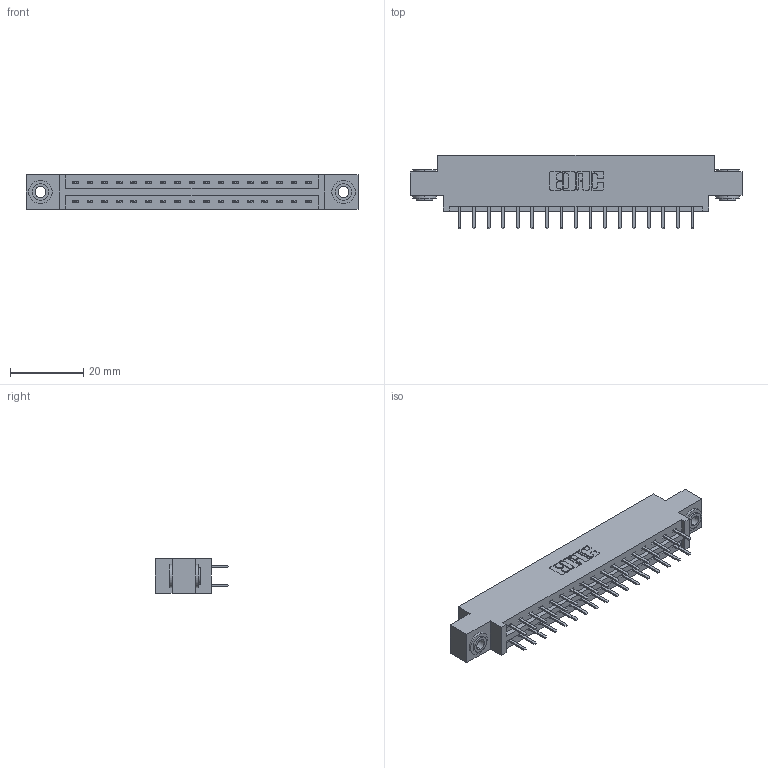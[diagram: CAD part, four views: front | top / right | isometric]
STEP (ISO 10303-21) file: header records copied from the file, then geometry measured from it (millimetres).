
FILE_DESCRIPTION (( 'STEP AP203' ), '1' );
FILE_NAME ('387-034-520-803.STEP', '2019-10-17T16:54:26', ( '' ), ( '' ), 'SwSTEP 2.0', 'SolidWorks 2016', '' );
FILE_SCHEMA (( 'CONFIG_CONTROL_DESIGN' ));
Length unit declared in the file: inch
Products named in the file (4): 387-034-520-803; 345-250-002_345-250-002-102; 345-292-001_345-293-120; 337 Part_0.170 Offset - 0.156 Dia-TH
Assembly tree (37 placements, depth 2):
  387-034-520-803
    337 Part_0.170 Offset - 0.156 Dia-TH
    345-292-001_345-293-120  x34
    345-250-002_345-250-002-102  x2
Bounding box: 90.37 x 20.02 x 9.4 mm (x, y, z)
Volume: 9078.4 mm3; surface area: 10309.9 mm2
Topology: 37 solids, 37 shells, 2128 faces, 6145 edges, 4002 vertices
Faces by surface type: plane 1444, cylinder 676, cone 8
Entity records: 17310 total; most frequent: CARTESIAN_POINT 2925, ORIENTED_EDGE 2842, DIRECTION 2555, EDGE_CURVE 1421, VECTOR 1265, LINE 1265, VERTEX_POINT 942, AXIS2_PLACEMENT_3D 645
